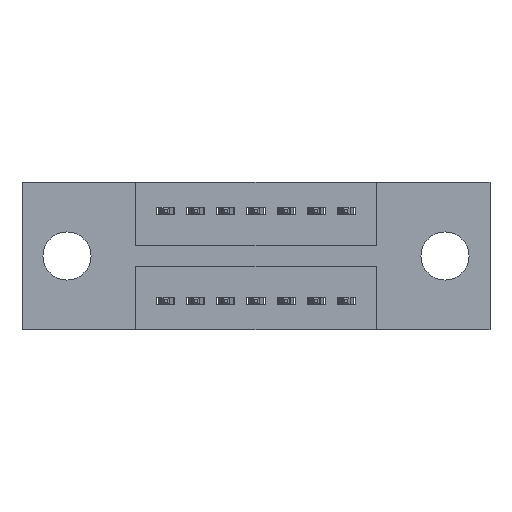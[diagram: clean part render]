
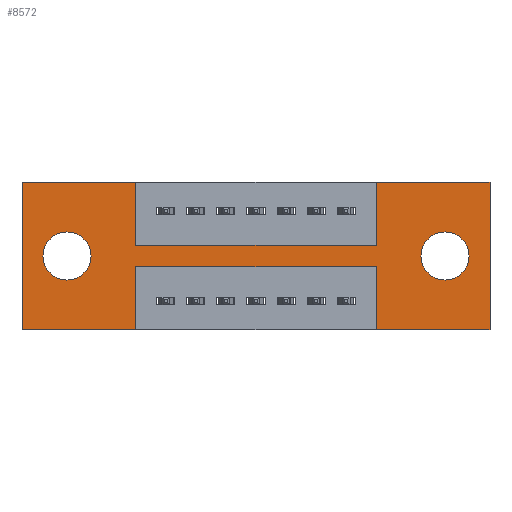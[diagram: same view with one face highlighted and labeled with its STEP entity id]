
A CAD part, front view. The second image highlights one B-rep face of the part: STEP entity #8572.
In plain terms, the highlighted planar face has unit normal (0, -1, 0).
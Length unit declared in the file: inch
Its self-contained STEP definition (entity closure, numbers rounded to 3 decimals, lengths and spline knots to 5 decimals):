
#29 = EDGE_LOOP ( 'NONE', ( #4906, #5427 ) ) ;
#44 = VERTEX_POINT ( 'NONE', #6212 ) ;
#87 = DIRECTION ( 'NONE',  ( 0., 0., -1. ) ) ;
#92 = DIRECTION ( 'NONE',  ( 1., 0., 0. ) ) ;
#97 = DIRECTION ( 'NONE',  ( 0., 1., 0. ) ) ;
#104 = CARTESIAN_POINT ( 'NONE',  ( 1.555, 0., 0. ) ) ;
#106 = EDGE_CURVE ( 'NONE', #44, #8850, #212, .T. ) ;
#110 = DIRECTION ( 'NONE',  ( -1., 0., 0. ) ) ;
#148 = CARTESIAN_POINT ( 'NONE',  ( 0., 0., 0. ) ) ;
#212 = CIRCLE ( 'NONE', #4134, 0.08 ) ;
#280 = EDGE_CURVE ( 'NONE', #1882, #3039, #2624, .T. ) ;
#327 = LINE ( 'NONE', #148, #5698 ) ;
#415 = EDGE_CURVE ( 'NONE', #1789, #4108, #8333, .T. ) ;
#546 = CARTESIAN_POINT ( 'NONE',  ( 0.3775, 0., -0.49 ) ) ;
#547 = DIRECTION ( 'NONE',  ( 0., 1., 0. ) ) ;
#673 = VERTEX_POINT ( 'NONE', #3506 ) ;
#738 = CARTESIAN_POINT ( 'NONE',  ( 0.3775, 0., -0.21 ) ) ;
#789 = EDGE_CURVE ( 'NONE', #6396, #673, #3075, .T. ) ;
#814 = DIRECTION ( 'NONE',  ( 0., 0., 1. ) ) ;
#856 = LINE ( 'NONE', #6337, #8088 ) ;
#897 = LINE ( 'NONE', #104, #2746 ) ;
#924 = CARTESIAN_POINT ( 'NONE',  ( 1.1775, 0., -0.28 ) ) ;
#978 = LINE ( 'NONE', #3093, #2739 ) ;
#979 = ORIENTED_EDGE ( 'NONE', *, *, #789, .F. ) ;
#1095 = DIRECTION ( 'NONE',  ( -1., 0., 0. ) ) ;
#1136 = VERTEX_POINT ( 'NONE', #546 ) ;
#1172 = CIRCLE ( 'NONE', #6493, 0.08 ) ;
#1187 = VECTOR ( 'NONE', #110, 39.37008 ) ;
#1232 = EDGE_CURVE ( 'NONE', #2007, #2709, #897, .T. ) ;
#1305 = CARTESIAN_POINT ( 'NONE',  ( 0.3775, 0., -0.21 ) ) ;
#1392 = FACE_OUTER_BOUND ( 'NONE', #6720, .T. ) ;
#1520 = ORIENTED_EDGE ( 'NONE', *, *, #4945, .F. ) ;
#1525 = CARTESIAN_POINT ( 'NONE',  ( 0.1495, 0., -0.245 ) ) ;
#1631 = CARTESIAN_POINT ( 'NONE',  ( 1.4055, 0., -0.325 ) ) ;
#1789 = VERTEX_POINT ( 'NONE', #3151 ) ;
#1882 = VERTEX_POINT ( 'NONE', #5182 ) ;
#1903 = CIRCLE ( 'NONE', #6754, 0.08 ) ;
#1969 = ORIENTED_EDGE ( 'NONE', *, *, #6942, .F. ) ;
#2007 = VERTEX_POINT ( 'NONE', #8871 ) ;
#2050 = ORIENTED_EDGE ( 'NONE', *, *, #4449, .F. ) ;
#2077 = LINE ( 'NONE', #5437, #7333 ) ;
#2086 = VECTOR ( 'NONE', #7274, 39.37008 ) ;
#2178 = DIRECTION ( 'NONE',  ( 1., 0., 0. ) ) ;
#2228 = CARTESIAN_POINT ( 'NONE',  ( 1.1775, 0., 0. ) ) ;
#2309 = CARTESIAN_POINT ( 'NONE',  ( 0., 0., 0. ) ) ;
#2336 = CARTESIAN_POINT ( 'NONE',  ( 1.4055, 0., -0.245 ) ) ;
#2373 = AXIS2_PLACEMENT_3D ( 'NONE', #3615, #97, #814 ) ;
#2560 = ORIENTED_EDGE ( 'NONE', *, *, #280, .F. ) ;
#2561 = DIRECTION ( 'NONE',  ( 0., 0., -1. ) ) ;
#2624 = LINE ( 'NONE', #5812, #2086 ) ;
#2709 = VERTEX_POINT ( 'NONE', #6537 ) ;
#2739 = VECTOR ( 'NONE', #3823, 39.37008 ) ;
#2746 = VECTOR ( 'NONE', #4366, 39.37008 ) ;
#2747 = DIRECTION ( 'NONE',  ( 0., 0., -1. ) ) ;
#2803 = LINE ( 'NONE', #1305, #8625 ) ;
#2856 = PLANE ( 'NONE',  #2889 ) ;
#2869 = ORIENTED_EDGE ( 'NONE', *, *, #3352, .T. ) ;
#2889 = AXIS2_PLACEMENT_3D ( 'NONE', #4293, #7801, #87 ) ;
#3030 = CARTESIAN_POINT ( 'NONE',  ( 0.3775, 0., 0. ) ) ;
#3039 = VERTEX_POINT ( 'NONE', #8745 ) ;
#3075 = LINE ( 'NONE', #6411, #1187 ) ;
#3093 = CARTESIAN_POINT ( 'NONE',  ( 0.3775, 0., -0.21 ) ) ;
#3133 = ORIENTED_EDGE ( 'NONE', *, *, #7767, .F. ) ;
#3146 = CARTESIAN_POINT ( 'NONE',  ( 0., 0., -0.49 ) ) ;
#3151 = CARTESIAN_POINT ( 'NONE',  ( 1.1775, 0., -0.21 ) ) ;
#3297 = ORIENTED_EDGE ( 'NONE', *, *, #1232, .F. ) ;
#3352 = EDGE_CURVE ( 'NONE', #8850, #44, #8308, .T. ) ;
#3385 = ORIENTED_EDGE ( 'NONE', *, *, #5317, .F. ) ;
#3448 = ORIENTED_EDGE ( 'NONE', *, *, #7826, .F. ) ;
#3506 = CARTESIAN_POINT ( 'NONE',  ( 0.3775, 0., -0.28 ) ) ;
#3615 = CARTESIAN_POINT ( 'NONE',  ( 0.1495, 0., -0.245 ) ) ;
#3635 = ORIENTED_EDGE ( 'NONE', *, *, #7125, .F. ) ;
#3646 = DIRECTION ( 'NONE',  ( 0., 1., 0. ) ) ;
#3742 = VERTEX_POINT ( 'NONE', #738 ) ;
#3823 = DIRECTION ( 'NONE',  ( 1., 0., 0. ) ) ;
#3864 = LINE ( 'NONE', #3146, #7253 ) ;
#3882 = DIRECTION ( 'NONE',  ( 0., 0., -1. ) ) ;
#3996 = CARTESIAN_POINT ( 'NONE',  ( 0.1495, 0., -0.165 ) ) ;
#4108 = VERTEX_POINT ( 'NONE', #2228 ) ;
#4134 = AXIS2_PLACEMENT_3D ( 'NONE', #1525, #3646, #7031 ) ;
#4293 = CARTESIAN_POINT ( 'NONE',  ( 0., 0., -0.49 ) ) ;
#4366 = DIRECTION ( 'NONE',  ( 0., 0., -1. ) ) ;
#4400 = LINE ( 'NONE', #2309, #8749 ) ;
#4449 = EDGE_CURVE ( 'NONE', #4108, #2007, #4400, .T. ) ;
#4655 = CARTESIAN_POINT ( 'NONE',  ( 1.1775, 0., -0.21 ) ) ;
#4886 = VERTEX_POINT ( 'NONE', #9066 ) ;
#4906 = ORIENTED_EDGE ( 'NONE', *, *, #6437, .T. ) ;
#4945 = EDGE_CURVE ( 'NONE', #4886, #6396, #856, .T. ) ;
#5133 = DIRECTION ( 'NONE',  ( 0., 1., 0. ) ) ;
#5146 = EDGE_LOOP ( 'NONE', ( #2869, #6764 ) ) ;
#5182 = CARTESIAN_POINT ( 'NONE',  ( 0., 0., -0.49 ) ) ;
#5293 = CARTESIAN_POINT ( 'NONE',  ( 0., 0., -0.49 ) ) ;
#5317 = EDGE_CURVE ( 'NONE', #6827, #3742, #2803, .T. ) ;
#5417 = VECTOR ( 'NONE', #5922, 39.37008 ) ;
#5427 = ORIENTED_EDGE ( 'NONE', *, *, #8861, .T. ) ;
#5437 = CARTESIAN_POINT ( 'NONE',  ( 0.3775, 0., -0.28 ) ) ;
#5598 = VERTEX_POINT ( 'NONE', #1631 ) ;
#5608 = CARTESIAN_POINT ( 'NONE',  ( 1.4055, 0., -0.165 ) ) ;
#5698 = VECTOR ( 'NONE', #92, 39.37008 ) ;
#5812 = CARTESIAN_POINT ( 'NONE',  ( 0., 0., 0. ) ) ;
#5922 = DIRECTION ( 'NONE',  ( -1., 0., 0. ) ) ;
#5937 = ORIENTED_EDGE ( 'NONE', *, *, #415, .F. ) ;
#6042 = VECTOR ( 'NONE', #7470, 39.37008 ) ;
#6173 = DIRECTION ( 'NONE',  ( 0., 0., -1. ) ) ;
#6212 = CARTESIAN_POINT ( 'NONE',  ( 0.1495, 0., -0.325 ) ) ;
#6286 = VERTEX_POINT ( 'NONE', #5608 ) ;
#6337 = CARTESIAN_POINT ( 'NONE',  ( 1.1775, 0., -0.28 ) ) ;
#6396 = VERTEX_POINT ( 'NONE', #924 ) ;
#6411 = CARTESIAN_POINT ( 'NONE',  ( 0.3775, 0., -0.28 ) ) ;
#6437 = EDGE_CURVE ( 'NONE', #6286, #5598, #1903, .T. ) ;
#6493 = AXIS2_PLACEMENT_3D ( 'NONE', #6838, #547, #6173 ) ;
#6537 = CARTESIAN_POINT ( 'NONE',  ( 1.555, 0., -0.49 ) ) ;
#6720 = EDGE_LOOP ( 'NONE', ( #5937, #3448, #3385, #3133, #2560, #1969, #3635, #979, #1520, #8888, #3297, #2050 ) ) ;
#6754 = AXIS2_PLACEMENT_3D ( 'NONE', #2336, #5133, #3882 ) ;
#6764 = ORIENTED_EDGE ( 'NONE', *, *, #106, .T. ) ;
#6827 = VERTEX_POINT ( 'NONE', #3030 ) ;
#6838 = CARTESIAN_POINT ( 'NONE',  ( 1.4055, 0., -0.245 ) ) ;
#6942 = EDGE_CURVE ( 'NONE', #1136, #1882, #8701, .T. ) ;
#7031 = DIRECTION ( 'NONE',  ( 0., 0., 1. ) ) ;
#7125 = EDGE_CURVE ( 'NONE', #673, #1136, #2077, .T. ) ;
#7253 = VECTOR ( 'NONE', #1095, 39.37008 ) ;
#7274 = DIRECTION ( 'NONE',  ( 0., 0., 1. ) ) ;
#7333 = VECTOR ( 'NONE', #2561, 39.37008 ) ;
#7458 = EDGE_CURVE ( 'NONE', #2709, #4886, #3864, .T. ) ;
#7470 = DIRECTION ( 'NONE',  ( 0., 0., 1. ) ) ;
#7536 = FACE_BOUND ( 'NONE', #29, .T. ) ;
#7674 = DIRECTION ( 'NONE',  ( 0., 0., 1. ) ) ;
#7767 = EDGE_CURVE ( 'NONE', #3039, #6827, #327, .T. ) ;
#7801 = DIRECTION ( 'NONE',  ( 0., -1., 0. ) ) ;
#7826 = EDGE_CURVE ( 'NONE', #3742, #1789, #978, .T. ) ;
#8088 = VECTOR ( 'NONE', #7674, 39.37008 ) ;
#8094 = FACE_BOUND ( 'NONE', #5146, .T. ) ;
#8308 = CIRCLE ( 'NONE', #2373, 0.08 ) ;
#8333 = LINE ( 'NONE', #4655, #6042 ) ;
#8572 = ADVANCED_FACE ( 'NONE', ( #7536, #8094, #1392 ), #2856, .T. ) ;
#8625 = VECTOR ( 'NONE', #2747, 39.37008 ) ;
#8701 = LINE ( 'NONE', #5293, #5417 ) ;
#8745 = CARTESIAN_POINT ( 'NONE',  ( 0., 0., 0. ) ) ;
#8749 = VECTOR ( 'NONE', #2178, 39.37008 ) ;
#8850 = VERTEX_POINT ( 'NONE', #3996 ) ;
#8861 = EDGE_CURVE ( 'NONE', #5598, #6286, #1172, .T. ) ;
#8871 = CARTESIAN_POINT ( 'NONE',  ( 1.555, 0., 0. ) ) ;
#8888 = ORIENTED_EDGE ( 'NONE', *, *, #7458, .F. ) ;
#9066 = CARTESIAN_POINT ( 'NONE',  ( 1.1775, 0., -0.49 ) ) ;
